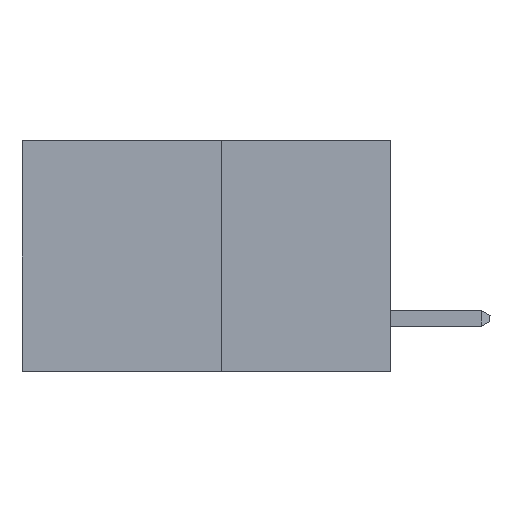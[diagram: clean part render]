
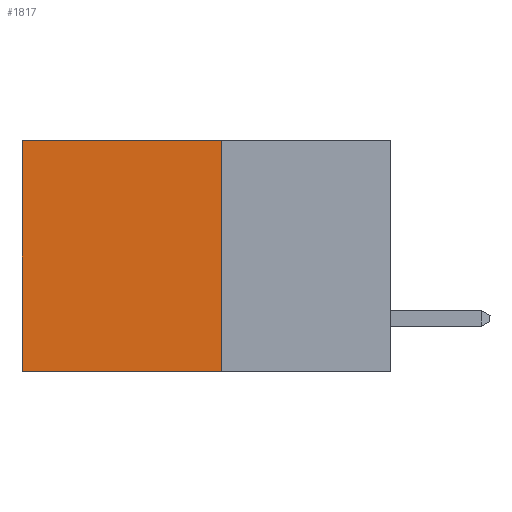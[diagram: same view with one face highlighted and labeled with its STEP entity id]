
A CAD part, left-side view. The second image highlights one B-rep face of the part: STEP entity #1817.
In plain terms, the highlighted planar face has unit normal (-1, 0, 0).
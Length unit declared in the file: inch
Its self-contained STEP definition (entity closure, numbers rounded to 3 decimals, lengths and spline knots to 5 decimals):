
#156 = CARTESIAN_POINT ( 'NONE',  ( 0.277, 0.27, -0.37 ) ) ;
#256 = VECTOR ( 'NONE', #3456, 39.37008 ) ;
#481 = PLANE ( 'NONE',  #3944 ) ;
#912 = VECTOR ( 'NONE', #5108, 39.37008 ) ;
#976 = DIRECTION ( 'NONE',  ( 0., 0., -1. ) ) ;
#1104 = DIRECTION ( 'NONE',  ( 1., 0., 0. ) ) ;
#1216 = LINE ( 'NONE', #4339, #912 ) ;
#1612 = VERTEX_POINT ( 'NONE', #5507 ) ;
#1817 = ADVANCED_FACE ( 'NONE', ( #2630 ), #481, .F. ) ;
#1866 = LINE ( 'NONE', #4997, #3729 ) ;
#2597 = LINE ( 'NONE', #3082, #256 ) ;
#2630 = FACE_OUTER_BOUND ( 'NONE', #6487, .T. ) ;
#3082 = CARTESIAN_POINT ( 'NONE',  ( 0.277, 0.27, -0.37 ) ) ;
#3091 = CARTESIAN_POINT ( 'NONE',  ( 0.277, 0.59, 0. ) ) ;
#3193 = ORIENTED_EDGE ( 'NONE', *, *, #3196, .F. ) ;
#3196 = EDGE_CURVE ( 'NONE', #1612, #7640, #2597, .T. ) ;
#3431 = ORIENTED_EDGE ( 'NONE', *, *, #8718, .T. ) ;
#3456 = DIRECTION ( 'NONE',  ( 0., 0., -1. ) ) ;
#3729 = VECTOR ( 'NONE', #7179, 39.37008 ) ;
#3794 = ORIENTED_EDGE ( 'NONE', *, *, #8466, .F. ) ;
#3944 = AXIS2_PLACEMENT_3D ( 'NONE', #156, #1104, #976 ) ;
#4339 = CARTESIAN_POINT ( 'NONE',  ( 0.277, 0.59, -0.37 ) ) ;
#4806 = CARTESIAN_POINT ( 'NONE',  ( 0.277, 0.27, -0.37 ) ) ;
#4997 = CARTESIAN_POINT ( 'NONE',  ( 0.277, 0.27, 0. ) ) ;
#5108 = DIRECTION ( 'NONE',  ( 0., 0., -1. ) ) ;
#5449 = ORIENTED_EDGE ( 'NONE', *, *, #7985, .T. ) ;
#5507 = CARTESIAN_POINT ( 'NONE',  ( 0.277, 0.27, 0. ) ) ;
#6292 = CARTESIAN_POINT ( 'NONE',  ( 0.277, 0.27, -0.37 ) ) ;
#6487 = EDGE_LOOP ( 'NONE', ( #5449, #3794, #3193, #3431 ) ) ;
#6970 = VERTEX_POINT ( 'NONE', #3091 ) ;
#7137 = CARTESIAN_POINT ( 'NONE',  ( 0.277, 0.59, -0.37 ) ) ;
#7179 = DIRECTION ( 'NONE',  ( 0., 1., 0. ) ) ;
#7306 = VECTOR ( 'NONE', #9005, 39.37008 ) ;
#7640 = VERTEX_POINT ( 'NONE', #4806 ) ;
#7808 = VERTEX_POINT ( 'NONE', #7137 ) ;
#7985 = EDGE_CURVE ( 'NONE', #6970, #7808, #1216, .T. ) ;
#8466 = EDGE_CURVE ( 'NONE', #7640, #7808, #9072, .T. ) ;
#8718 = EDGE_CURVE ( 'NONE', #1612, #6970, #1866, .T. ) ;
#9005 = DIRECTION ( 'NONE',  ( 0., 1., 0. ) ) ;
#9072 = LINE ( 'NONE', #6292, #7306 ) ;
